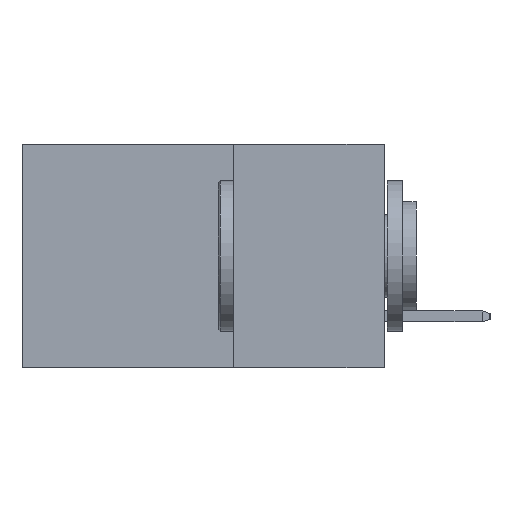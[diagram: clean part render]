
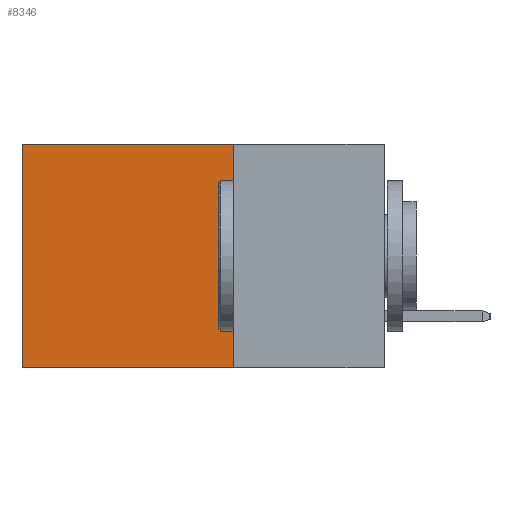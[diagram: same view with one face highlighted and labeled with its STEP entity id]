
A CAD part, left-side view. The second image highlights one B-rep face of the part: STEP entity #8346.
In plain terms, the highlighted planar face has unit normal (-1, 0, 0).
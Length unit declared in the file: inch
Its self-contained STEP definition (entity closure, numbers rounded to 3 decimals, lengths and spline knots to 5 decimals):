
#46 = VECTOR ( 'NONE', #22408, 39.37008 ) ;
#125 = VERTEX_POINT ( 'NONE', #4266 ) ;
#492 = ORIENTED_EDGE ( 'NONE', *, *, #594, .F. ) ;
#594 = EDGE_CURVE ( 'NONE', #125, #5041, #14484, .T. ) ;
#720 = ORIENTED_EDGE ( 'NONE', *, *, #18568, .T. ) ;
#2075 = DIRECTION ( 'NONE',  ( 0., 0., -1. ) ) ;
#2103 = CARTESIAN_POINT ( 'NONE',  ( 0.298, 0.6, 0. ) ) ;
#2693 = CARTESIAN_POINT ( 'NONE',  ( 0.298, 0.25, 0. ) ) ;
#3141 = VECTOR ( 'NONE', #12695, 39.37008 ) ;
#4266 = CARTESIAN_POINT ( 'NONE',  ( 0.298, 0.25, 0. ) ) ;
#5041 = VERTEX_POINT ( 'NONE', #18837 ) ;
#6095 = FACE_OUTER_BOUND ( 'NONE', #8487, .T. ) ;
#7184 = DIRECTION ( 'NONE',  ( 0., 0., -1. ) ) ;
#7981 = VERTEX_POINT ( 'NONE', #13203 ) ;
#8346 = ADVANCED_FACE ( 'NONE', ( #6095 ), #12459, .F. ) ;
#8475 = ORIENTED_EDGE ( 'NONE', *, *, #14497, .T. ) ;
#8487 = EDGE_LOOP ( 'NONE', ( #8475, #10050, #492, #720 ) ) ;
#10050 = ORIENTED_EDGE ( 'NONE', *, *, #10999, .F. ) ;
#10129 = LINE ( 'NONE', #20709, #46 ) ;
#10694 = CARTESIAN_POINT ( 'NONE',  ( 0.298, 0.25, 0. ) ) ;
#10999 = EDGE_CURVE ( 'NONE', #5041, #15322, #10129, .T. ) ;
#11743 = CARTESIAN_POINT ( 'NONE',  ( 0.298, 0.25, 0. ) ) ;
#12459 = PLANE ( 'NONE',  #14366 ) ;
#12585 = LINE ( 'NONE', #2103, #3141 ) ;
#12695 = DIRECTION ( 'NONE',  ( 0., 0., -1. ) ) ;
#13203 = CARTESIAN_POINT ( 'NONE',  ( 0.298, 0.6, 0. ) ) ;
#13486 = DIRECTION ( 'NONE',  ( 0., 1., 0. ) ) ;
#14366 = AXIS2_PLACEMENT_3D ( 'NONE', #10694, #17709, #7184 ) ;
#14383 = VECTOR ( 'NONE', #13486, 39.37008 ) ;
#14484 = LINE ( 'NONE', #2693, #22557 ) ;
#14497 = EDGE_CURVE ( 'NONE', #7981, #15322, #12585, .T. ) ;
#15322 = VERTEX_POINT ( 'NONE', #21923 ) ;
#17709 = DIRECTION ( 'NONE',  ( 1., 0., 0. ) ) ;
#18568 = EDGE_CURVE ( 'NONE', #125, #7981, #20071, .T. ) ;
#18837 = CARTESIAN_POINT ( 'NONE',  ( 0.298, 0.25, -0.37 ) ) ;
#20071 = LINE ( 'NONE', #11743, #14383 ) ;
#20709 = CARTESIAN_POINT ( 'NONE',  ( 0.298, 0.25, -0.37 ) ) ;
#21923 = CARTESIAN_POINT ( 'NONE',  ( 0.298, 0.6, -0.37 ) ) ;
#22408 = DIRECTION ( 'NONE',  ( 0., 1., 0. ) ) ;
#22557 = VECTOR ( 'NONE', #2075, 39.37008 ) ;
